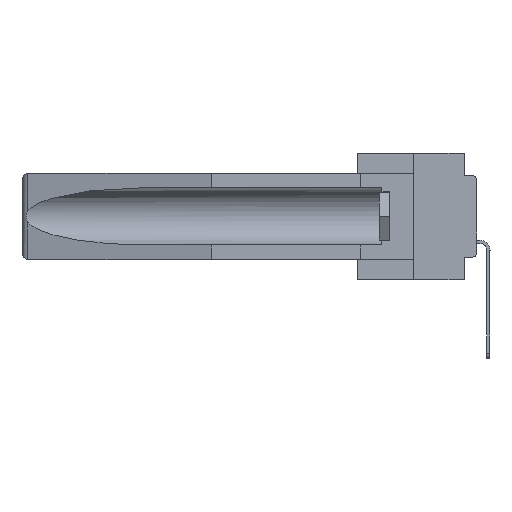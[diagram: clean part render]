
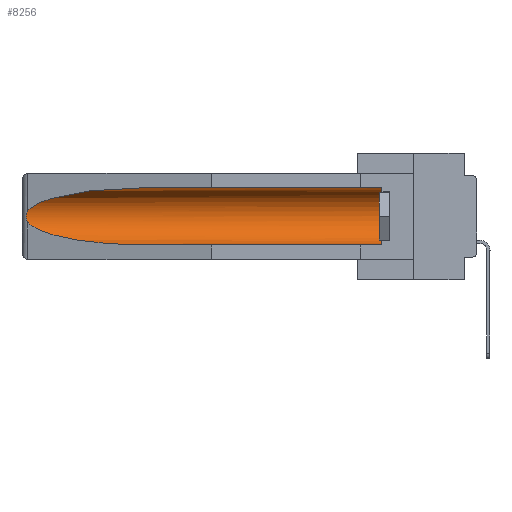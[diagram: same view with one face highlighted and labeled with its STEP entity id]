
A CAD part, left-side view. The second image highlights one B-rep face of the part: STEP entity #8256.
In plain terms, the highlighted cylindrical face has radius 2.857 mm (diameter 5.715 mm), a partial arc.
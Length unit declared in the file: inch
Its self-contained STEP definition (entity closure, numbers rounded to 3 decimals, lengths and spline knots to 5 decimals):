
#127 = ORIENTED_EDGE ( 'NONE', *, *, #31029, .T. ) ;
#393 = ORIENTED_EDGE ( 'NONE', *, *, #7449, .T. ) ;
#832 = AXIS2_PLACEMENT_3D ( 'NONE', #1678, #17385, #7025 ) ;
#911 = ORIENTED_EDGE ( 'NONE', *, *, #20548, .F. ) ;
#1247 = VERTEX_POINT ( 'NONE', #30103 ) ;
#1294 = CARTESIAN_POINT ( 'NONE',  ( 0.155, 0.126, -0.059 ) ) ;
#1470 = CARTESIAN_POINT ( 'NONE',  ( 0.26537, 1.52718, -0.14972 ) ) ;
#1678 = CARTESIAN_POINT ( 'NONE',  ( 0.155, -0.30754, -0.1715 ) ) ;
#2221 = CARTESIAN_POINT ( 'NONE',  ( 0.21114, 1.30732, -0.284 ) ) ;
#2251 = CARTESIAN_POINT ( 'NONE',  ( 0.155, -0.30754, -0.284 ) ) ;
#4128 = LINE ( 'NONE', #15866, #8650 ) ;
#5030 = VERTEX_POINT ( 'NONE', #8938 ) ;
#5637 = FACE_OUTER_BOUND ( 'NONE', #28126, .T. ) ;
#5787 = CARTESIAN_POINT ( 'NONE',  ( 0.21114, 1.30732, -0.059 ) ) ;
#5796 = CARTESIAN_POINT ( 'NONE',  ( 0.26537, 1.52718, -0.19328 ) ) ;
#5907 = CARTESIAN_POINT ( 'NONE',  ( 0.26654, 1.53092, -0.15636 ) ) ;
#6037 = CARTESIAN_POINT ( 'NONE',  ( 0.26597, 1.52961, -0.15275 ) ) ;
#7025 = DIRECTION ( 'NONE',  ( 0., 0., 1. ) ) ;
#7041 =( BOUNDED_CURVE ( )  B_SPLINE_CURVE ( 3, ( #18050, #28739, #2221, #9992 ),
 .UNSPECIFIED., .F., .F. ) 
 B_SPLINE_CURVE_WITH_KNOTS ( ( 4, 4 ),
 ( 0.1948, 1.5708 ),
 .UNSPECIFIED. ) 
 CURVE ( )  GEOMETRIC_REPRESENTATION_ITEM ( )  RATIONAL_B_SPLINE_CURVE ( ( 1., 0.848, 0.848, 1. ) ) 
 REPRESENTATION_ITEM ( '' )  );
#7422 = CIRCLE ( 'NONE', #20964, 0.1125 ) ;
#7449 = EDGE_CURVE ( 'NONE', #19807, #1247, #18240, .T. ) ;
#8256 = ADVANCED_FACE ( 'NONE', ( #5637 ), #25023, .F. ) ;
#8650 = VECTOR ( 'NONE', #16197, 39.37008 ) ;
#8938 = CARTESIAN_POINT ( 'NONE',  ( 0.155, 1.07973, -0.059 ) ) ;
#9992 = CARTESIAN_POINT ( 'NONE',  ( 0.155, 1.07973, -0.284 ) ) ;
#10324 = EDGE_CURVE ( 'NONE', #1247, #25538, #7041, .T. ) ;
#13762 = CARTESIAN_POINT ( 'NONE',  ( 0.2673, 1.5327, -0.16383 ) ) ;
#13864 = CARTESIAN_POINT ( 'NONE',  ( 0.26537, 1.52718, -0.14972 ) ) ;
#15866 = CARTESIAN_POINT ( 'NONE',  ( 0.155, -0.30754, -0.059 ) ) ;
#16051 = DIRECTION ( 'NONE',  ( 0., 0., 1. ) ) ;
#16168 = CARTESIAN_POINT ( 'NONE',  ( 0.155, 0.126, -0.1715 ) ) ;
#16197 = DIRECTION ( 'NONE',  ( 0., 1., 0. ) ) ;
#16289 = ORIENTED_EDGE ( 'NONE', *, *, #10324, .T. ) ;
#16936 = EDGE_CURVE ( 'NONE', #5030, #19807, #23903, .T. ) ;
#17385 = DIRECTION ( 'NONE',  ( 0., 1., 0. ) ) ;
#18050 = CARTESIAN_POINT ( 'NONE',  ( 0.26537, 1.52718, -0.19328 ) ) ;
#18240 = B_SPLINE_CURVE_WITH_KNOTS ( 'NONE', 3,
 ( #19171, #6037, #5907, #13762, #32171, #24353, #24468, #32507, #27108, #5796 ),
 .UNSPECIFIED., .F., .F.,
 ( 4, 2, 2, 2, 4 ),
 ( 0., 0.00029, 0.00058, 0.00087, 0.00117 ),
 .UNSPECIFIED. ) ;
#18572 = LINE ( 'NONE', #2251, #24332 ) ;
#19171 = CARTESIAN_POINT ( 'NONE',  ( 0.26537, 1.52718, -0.14972 ) ) ;
#19807 = VERTEX_POINT ( 'NONE', #1470 ) ;
#20548 = EDGE_CURVE ( 'NONE', #23878, #25538, #18572, .T. ) ;
#20964 = AXIS2_PLACEMENT_3D ( 'NONE', #16168, #26530, #16051 ) ;
#23878 = VERTEX_POINT ( 'NONE', #31004 ) ;
#23903 =( BOUNDED_CURVE ( )  B_SPLINE_CURVE ( 3, ( #24341, #5787, #32049, #13864 ),
 .UNSPECIFIED., .F., .F. ) 
 B_SPLINE_CURVE_WITH_KNOTS ( ( 4, 4 ),
 ( 4.71239, 6.08839 ),
 .UNSPECIFIED. ) 
 CURVE ( )  GEOMETRIC_REPRESENTATION_ITEM ( )  RATIONAL_B_SPLINE_CURVE ( ( 1., 0.848, 0.848, 1. ) ) 
 REPRESENTATION_ITEM ( '' )  );
#24105 = ORIENTED_EDGE ( 'NONE', *, *, #16936, .T. ) ;
#24332 = VECTOR ( 'NONE', #31418, 39.37008 ) ;
#24341 = CARTESIAN_POINT ( 'NONE',  ( 0.155, 1.07973, -0.059 ) ) ;
#24353 = CARTESIAN_POINT ( 'NONE',  ( 0.2675, 1.53308, -0.17534 ) ) ;
#24468 = CARTESIAN_POINT ( 'NONE',  ( 0.2673, 1.53269, -0.17917 ) ) ;
#25023 = CYLINDRICAL_SURFACE ( 'NONE', #832, 0.1125 ) ;
#25538 = VERTEX_POINT ( 'NONE', #25823 ) ;
#25823 = CARTESIAN_POINT ( 'NONE',  ( 0.155, 1.07973, -0.284 ) ) ;
#26530 = DIRECTION ( 'NONE',  ( 0., -1., 0. ) ) ;
#27108 = CARTESIAN_POINT ( 'NONE',  ( 0.26597, 1.5296, -0.19026 ) ) ;
#27556 = VERTEX_POINT ( 'NONE', #1294 ) ;
#28126 = EDGE_LOOP ( 'NONE', ( #24105, #393, #16289, #911, #32322, #127 ) ) ;
#28739 = CARTESIAN_POINT ( 'NONE',  ( 0.25451, 1.48313, -0.24835 ) ) ;
#29736 = EDGE_CURVE ( 'NONE', #23878, #27556, #7422, .T. ) ;
#30103 = CARTESIAN_POINT ( 'NONE',  ( 0.26537, 1.52718, -0.19328 ) ) ;
#31004 = CARTESIAN_POINT ( 'NONE',  ( 0.155, 0.126, -0.284 ) ) ;
#31029 = EDGE_CURVE ( 'NONE', #27556, #5030, #4128, .T. ) ;
#31418 = DIRECTION ( 'NONE',  ( 0., 1., 0. ) ) ;
#32049 = CARTESIAN_POINT ( 'NONE',  ( 0.25451, 1.48313, -0.09465 ) ) ;
#32171 = CARTESIAN_POINT ( 'NONE',  ( 0.2675, 1.53308, -0.16763 ) ) ;
#32322 = ORIENTED_EDGE ( 'NONE', *, *, #29736, .T. ) ;
#32507 = CARTESIAN_POINT ( 'NONE',  ( 0.26655, 1.53094, -0.18657 ) ) ;
